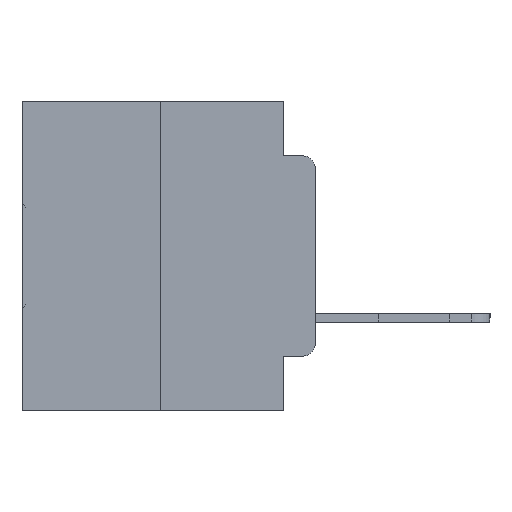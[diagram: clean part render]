
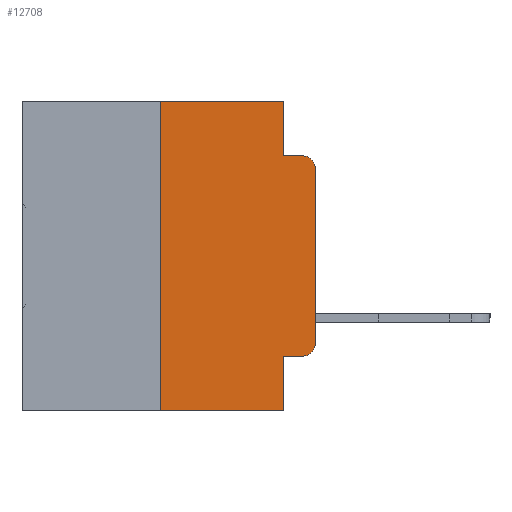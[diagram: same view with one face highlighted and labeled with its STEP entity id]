
A CAD part, left-side view. The second image highlights one B-rep face of the part: STEP entity #12708.
In plain terms, the highlighted planar face has unit normal (-1, 0, 0).
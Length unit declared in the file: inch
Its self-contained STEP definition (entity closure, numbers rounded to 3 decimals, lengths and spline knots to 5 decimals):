
#495 = ORIENTED_EDGE ( 'NONE', *, *, #9267, .F. ) ;
#544 = DIRECTION ( 'NONE',  ( 0., 0., -1. ) ) ;
#724 = ORIENTED_EDGE ( 'NONE', *, *, #30095, .F. ) ;
#727 = LINE ( 'NONE', #955, #6538 ) ;
#847 = ORIENTED_EDGE ( 'NONE', *, *, #12979, .T. ) ;
#877 = CARTESIAN_POINT ( 'NONE',  ( 0., 0.02, -0.1085 ) ) ;
#879 = ORIENTED_EDGE ( 'NONE', *, *, #24206, .F. ) ;
#930 = CARTESIAN_POINT ( 'NONE',  ( 0., 0.051, -0.0885 ) ) ;
#955 = CARTESIAN_POINT ( 'NONE',  ( 0., 0.473, -0.5 ) ) ;
#1062 = LINE ( 'NONE', #3746, #19005 ) ;
#1918 = AXIS2_PLACEMENT_3D ( 'NONE', #877, #17910, #3382 ) ;
#2378 = CARTESIAN_POINT ( 'NONE',  ( 0., 0., -0.3915 ) ) ;
#3382 = DIRECTION ( 'NONE',  ( 0., 0., -1. ) ) ;
#3746 = CARTESIAN_POINT ( 'NONE',  ( 0., 0.051, -0.4115 ) ) ;
#5139 = ORIENTED_EDGE ( 'NONE', *, *, #7105, .F. ) ;
#5522 = VERTEX_POINT ( 'NONE', #2378 ) ;
#6478 = VERTEX_POINT ( 'NONE', #23626 ) ;
#6538 = VECTOR ( 'NONE', #8265, 39.37008 ) ;
#6558 = DIRECTION ( 'NONE',  ( 0., -1., 0. ) ) ;
#6815 = VERTEX_POINT ( 'NONE', #22561 ) ;
#7053 = ORIENTED_EDGE ( 'NONE', *, *, #25201, .T. ) ;
#7105 = EDGE_CURVE ( 'NONE', #25213, #13793, #14843, .T. ) ;
#7803 = VECTOR ( 'NONE', #6558, 39.37008 ) ;
#8265 = DIRECTION ( 'NONE',  ( 0., -1., 0. ) ) ;
#8283 = CARTESIAN_POINT ( 'NONE',  ( 0., 0.25, -0.5 ) ) ;
#8291 = CARTESIAN_POINT ( 'NONE',  ( 0., 0.051, 0. ) ) ;
#8389 = VECTOR ( 'NONE', #26323, 39.37008 ) ;
#9267 = EDGE_CURVE ( 'NONE', #21349, #19079, #28248, .T. ) ;
#11175 = ORIENTED_EDGE ( 'NONE', *, *, #26967, .T. ) ;
#11589 = CARTESIAN_POINT ( 'NONE',  ( 0., 0.25, 0. ) ) ;
#12066 = CARTESIAN_POINT ( 'NONE',  ( 0., 0.051, 0. ) ) ;
#12708 = ADVANCED_FACE ( 'NONE', ( #21148 ), #29967, .F. ) ;
#12810 = CARTESIAN_POINT ( 'NONE',  ( 0., 0.051, 0. ) ) ;
#12979 = EDGE_CURVE ( 'NONE', #5522, #6478, #31539, .T. ) ;
#13119 = CARTESIAN_POINT ( 'NONE',  ( 0., 0.473, 0. ) ) ;
#13184 = EDGE_CURVE ( 'NONE', #16801, #18561, #14594, .T. ) ;
#13665 = DIRECTION ( 'NONE',  ( 0., 0., 1. ) ) ;
#13793 = VERTEX_POINT ( 'NONE', #24181 ) ;
#13812 = VECTOR ( 'NONE', #29299, 39.37008 ) ;
#13830 = VERTEX_POINT ( 'NONE', #19383 ) ;
#14234 = LINE ( 'NONE', #16062, #7803 ) ;
#14275 = CARTESIAN_POINT ( 'NONE',  ( 0., 0.02, -0.3915 ) ) ;
#14594 = LINE ( 'NONE', #12066, #13812 ) ;
#14843 = LINE ( 'NONE', #11589, #8389 ) ;
#15183 = DIRECTION ( 'NONE',  ( 1., 0., 0. ) ) ;
#16062 = CARTESIAN_POINT ( 'NONE',  ( 0., 0.051, -0.0885 ) ) ;
#16698 = DIRECTION ( 'NONE',  ( 0., 0., -1. ) ) ;
#16801 = VERTEX_POINT ( 'NONE', #27726 ) ;
#16902 = ORIENTED_EDGE ( 'NONE', *, *, #13184, .F. ) ;
#17910 = DIRECTION ( 'NONE',  ( -1., 0., 0. ) ) ;
#18000 = DIRECTION ( 'NONE',  ( 0., -1., 0. ) ) ;
#18206 = CIRCLE ( 'NONE', #20692, 0.02 ) ;
#18231 = ORIENTED_EDGE ( 'NONE', *, *, #21713, .T. ) ;
#18561 = VERTEX_POINT ( 'NONE', #28215 ) ;
#19005 = VECTOR ( 'NONE', #20794, 39.37008 ) ;
#19079 = VERTEX_POINT ( 'NONE', #930 ) ;
#19383 = CARTESIAN_POINT ( 'NONE',  ( 0., 0.02, -0.4115 ) ) ;
#20401 = VECTOR ( 'NONE', #18000, 39.37008 ) ;
#20692 = AXIS2_PLACEMENT_3D ( 'NONE', #14275, #31493, #16698 ) ;
#20794 = DIRECTION ( 'NONE',  ( 0., -1., 0. ) ) ;
#21148 = FACE_OUTER_BOUND ( 'NONE', #31777, .T. ) ;
#21349 = VERTEX_POINT ( 'NONE', #12810 ) ;
#21667 = VECTOR ( 'NONE', #25544, 39.37008 ) ;
#21713 = EDGE_CURVE ( 'NONE', #13830, #5522, #18206, .T. ) ;
#22521 = CARTESIAN_POINT ( 'NONE',  ( 0., 0.473, 0. ) ) ;
#22561 = CARTESIAN_POINT ( 'NONE',  ( 0., 0.02, -0.0885 ) ) ;
#23466 = CARTESIAN_POINT ( 'NONE',  ( 0., 0., 0. ) ) ;
#23626 = CARTESIAN_POINT ( 'NONE',  ( 0., 0., -0.1085 ) ) ;
#24181 = CARTESIAN_POINT ( 'NONE',  ( 0., 0.25, 0. ) ) ;
#24206 = EDGE_CURVE ( 'NONE', #19079, #6815, #14234, .T. ) ;
#25011 = VECTOR ( 'NONE', #13665, 39.37008 ) ;
#25201 = EDGE_CURVE ( 'NONE', #6478, #6815, #25741, .T. ) ;
#25213 = VERTEX_POINT ( 'NONE', #8283 ) ;
#25239 = ORIENTED_EDGE ( 'NONE', *, *, #27698, .T. ) ;
#25544 = DIRECTION ( 'NONE',  ( 0., 0., -1. ) ) ;
#25741 = CIRCLE ( 'NONE', #1918, 0.02 ) ;
#26323 = DIRECTION ( 'NONE',  ( 0., 0., 1. ) ) ;
#26967 = EDGE_CURVE ( 'NONE', #25213, #18561, #727, .T. ) ;
#27015 = LINE ( 'NONE', #13119, #20401 ) ;
#27698 = EDGE_CURVE ( 'NONE', #16801, #13830, #1062, .T. ) ;
#27726 = CARTESIAN_POINT ( 'NONE',  ( 0., 0.051, -0.4115 ) ) ;
#28215 = CARTESIAN_POINT ( 'NONE',  ( 0., 0.051, -0.5 ) ) ;
#28248 = LINE ( 'NONE', #8291, #21667 ) ;
#29299 = DIRECTION ( 'NONE',  ( 0., 0., -1. ) ) ;
#29462 = AXIS2_PLACEMENT_3D ( 'NONE', #22521, #15183, #544 ) ;
#29967 = PLANE ( 'NONE',  #29462 ) ;
#30095 = EDGE_CURVE ( 'NONE', #13793, #21349, #27015, .T. ) ;
#31493 = DIRECTION ( 'NONE',  ( -1., 0., 0. ) ) ;
#31539 = LINE ( 'NONE', #23466, #25011 ) ;
#31777 = EDGE_LOOP ( 'NONE', ( #847, #7053, #879, #495, #724, #5139, #11175, #16902, #25239, #18231 ) ) ;
